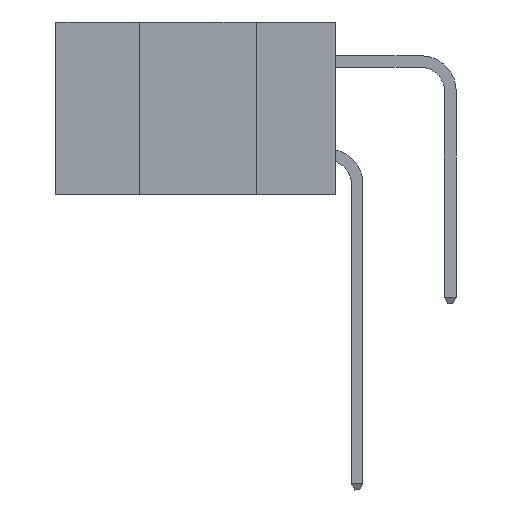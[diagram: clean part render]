
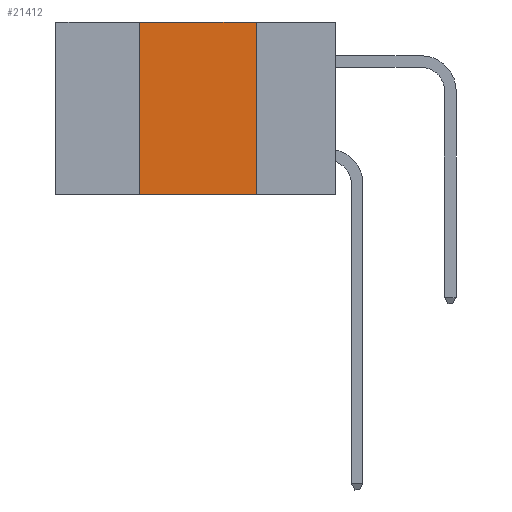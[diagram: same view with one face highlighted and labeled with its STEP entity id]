
A CAD part, left-side view. The second image highlights one B-rep face of the part: STEP entity #21412.
In plain terms, the highlighted planar face has unit normal (-1, 0, 0).
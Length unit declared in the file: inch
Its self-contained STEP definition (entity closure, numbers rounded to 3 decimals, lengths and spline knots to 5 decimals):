
#264 = CARTESIAN_POINT ( 'NONE',  ( 0., 0.17, 0. ) ) ;
#2279 = DIRECTION ( 'NONE',  ( 0., -1., 0. ) ) ;
#2577 = ORIENTED_EDGE ( 'NONE', *, *, #5658, .F. ) ;
#3007 = DIRECTION ( 'NONE',  ( 0., 0., 1. ) ) ;
#3154 = CARTESIAN_POINT ( 'NONE',  ( 0., 0.6, 0. ) ) ;
#3948 = EDGE_CURVE ( 'NONE', #16468, #18657, #10470, .T. ) ;
#4884 = DIRECTION ( 'NONE',  ( 0., 0., -1. ) ) ;
#5142 = LINE ( 'NONE', #14180, #9162 ) ;
#5658 = EDGE_CURVE ( 'NONE', #21225, #10169, #8383, .T. ) ;
#7306 = VECTOR ( 'NONE', #3007, 39.37008 ) ;
#7515 = EDGE_LOOP ( 'NONE', ( #11463, #10407, #2577, #19383 ) ) ;
#7996 = VECTOR ( 'NONE', #13143, 39.37008 ) ;
#8383 = LINE ( 'NONE', #14861, #7306 ) ;
#9162 = VECTOR ( 'NONE', #2279, 39.37008 ) ;
#9775 = CARTESIAN_POINT ( 'NONE',  ( 0., 0.6, -0.37 ) ) ;
#9827 = CARTESIAN_POINT ( 'NONE',  ( 0., 0.42, 0. ) ) ;
#10169 = VERTEX_POINT ( 'NONE', #9827 ) ;
#10407 = ORIENTED_EDGE ( 'NONE', *, *, #15631, .F. ) ;
#10470 = LINE ( 'NONE', #16967, #14381 ) ;
#11463 = ORIENTED_EDGE ( 'NONE', *, *, #3948, .F. ) ;
#12524 = LINE ( 'NONE', #9775, #7996 ) ;
#13143 = DIRECTION ( 'NONE',  ( 0., -1., 0. ) ) ;
#13350 = PLANE ( 'NONE',  #15548 ) ;
#14180 = CARTESIAN_POINT ( 'NONE',  ( 0., 0.6, 0. ) ) ;
#14381 = VECTOR ( 'NONE', #16428, 39.37008 ) ;
#14520 = CARTESIAN_POINT ( 'NONE',  ( 0., 0.42, -0.37 ) ) ;
#14861 = CARTESIAN_POINT ( 'NONE',  ( 0., 0.42, 0. ) ) ;
#15003 = DIRECTION ( 'NONE',  ( 1., 0., 0. ) ) ;
#15548 = AXIS2_PLACEMENT_3D ( 'NONE', #3154, #15003, #4884 ) ;
#15631 = EDGE_CURVE ( 'NONE', #10169, #16468, #5142, .T. ) ;
#16428 = DIRECTION ( 'NONE',  ( 0., 0., -1. ) ) ;
#16468 = VERTEX_POINT ( 'NONE', #264 ) ;
#16967 = CARTESIAN_POINT ( 'NONE',  ( 0., 0.17, 0. ) ) ;
#17936 = CARTESIAN_POINT ( 'NONE',  ( 0., 0.17, -0.37 ) ) ;
#18657 = VERTEX_POINT ( 'NONE', #17936 ) ;
#19383 = ORIENTED_EDGE ( 'NONE', *, *, #20663, .T. ) ;
#19882 = FACE_OUTER_BOUND ( 'NONE', #7515, .T. ) ;
#20663 = EDGE_CURVE ( 'NONE', #21225, #18657, #12524, .T. ) ;
#21225 = VERTEX_POINT ( 'NONE', #14520 ) ;
#21412 = ADVANCED_FACE ( 'NONE', ( #19882 ), #13350, .F. ) ;
